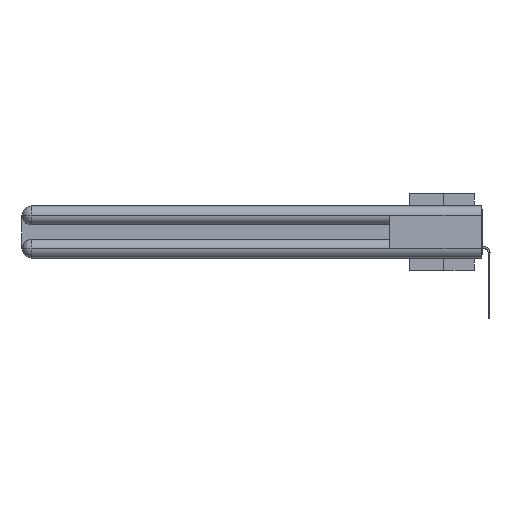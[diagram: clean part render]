
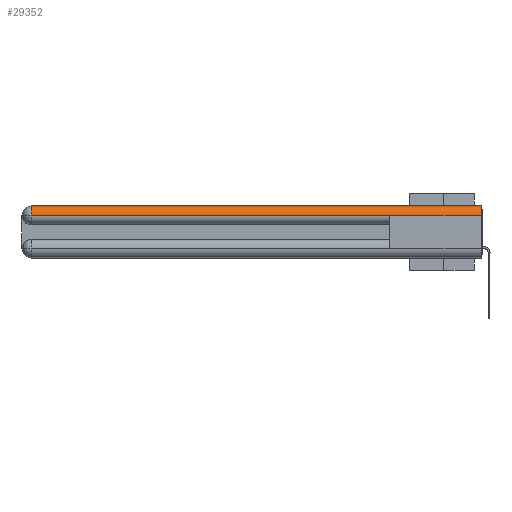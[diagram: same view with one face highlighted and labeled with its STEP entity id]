
A CAD part, left-side view. The second image highlights one B-rep face of the part: STEP entity #29352.
In plain terms, the highlighted cylindrical face has radius 1.562 mm (diameter 3.124 mm), a partial arc.
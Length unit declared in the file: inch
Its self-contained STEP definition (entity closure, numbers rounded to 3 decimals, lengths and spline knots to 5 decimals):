
#636 = LINE ( 'NONE', #3860, #15750 ) ;
#1578 = DIRECTION ( 'NONE',  ( 0., 0., 1. ) ) ;
#1835 = AXIS2_PLACEMENT_3D ( 'NONE', #13477, #21405, #1578 ) ;
#2423 = EDGE_LOOP ( 'NONE', ( #30328, #17633, #7823, #13776, #29750 ) ) ;
#3426 = DIRECTION ( 'NONE',  ( 1., 0., 0. ) ) ;
#3727 = CARTESIAN_POINT ( 'NONE',  ( 0., 3., -0.0615 ) ) ;
#3860 = CARTESIAN_POINT ( 'NONE',  ( 0.0615, 0., 0. ) ) ;
#4786 = VECTOR ( 'NONE', #35011, 39.37008 ) ;
#6468 = VECTOR ( 'NONE', #12490, 39.37008 ) ;
#6993 = VERTEX_POINT ( 'NONE', #33838 ) ;
#7823 = ORIENTED_EDGE ( 'NONE', *, *, #29557, .T. ) ;
#9452 = CARTESIAN_POINT ( 'NONE',  ( 0.0615, 0., -0.0615 ) ) ;
#10707 = CARTESIAN_POINT ( 'NONE',  ( 0., 2.94, -0.0615 ) ) ;
#12222 = LINE ( 'NONE', #3727, #4786 ) ;
#12490 = DIRECTION ( 'NONE',  ( 0., 1., 0. ) ) ;
#13162 = CIRCLE ( 'NONE', #34197, 0.0615 ) ;
#13477 = CARTESIAN_POINT ( 'NONE',  ( 0.0615, 2.94, -0.0615 ) ) ;
#13558 = VERTEX_POINT ( 'NONE', #17473 ) ;
#13776 = ORIENTED_EDGE ( 'NONE', *, *, #15268, .F. ) ;
#15144 = LINE ( 'NONE', #35475, #6468 ) ;
#15268 = EDGE_CURVE ( 'NONE', #6993, #36753, #15144, .T. ) ;
#15746 = DIRECTION ( 'NONE',  ( 0., -1., 0. ) ) ;
#15750 = VECTOR ( 'NONE', #15746, 39.37008 ) ;
#16899 = CIRCLE ( 'NONE', #1835, 0.0615 ) ;
#17440 = AXIS2_PLACEMENT_3D ( 'NONE', #26167, #29166, #17526 ) ;
#17473 = CARTESIAN_POINT ( 'NONE',  ( 0.0615, 0., 0. ) ) ;
#17526 = DIRECTION ( 'NONE',  ( 0., 0., 1. ) ) ;
#17633 = ORIENTED_EDGE ( 'NONE', *, *, #36425, .T. ) ;
#20985 = CARTESIAN_POINT ( 'NONE',  ( 0., 0.6, -0.0615 ) ) ;
#21405 = DIRECTION ( 'NONE',  ( 0., -1., 0. ) ) ;
#25004 = VERTEX_POINT ( 'NONE', #31355 ) ;
#25607 = CYLINDRICAL_SURFACE ( 'NONE', #17440, 0.0615 ) ;
#26167 = CARTESIAN_POINT ( 'NONE',  ( 0.0615, 0., -0.0615 ) ) ;
#29166 = DIRECTION ( 'NONE',  ( 0., 1., 0. ) ) ;
#29352 = ADVANCED_FACE ( 'NONE', ( #31610 ), #25607, .T. ) ;
#29557 = EDGE_CURVE ( 'NONE', #33645, #36753, #12222, .T. ) ;
#29750 = ORIENTED_EDGE ( 'NONE', *, *, #32968, .F. ) ;
#30328 = ORIENTED_EDGE ( 'NONE', *, *, #35737, .F. ) ;
#31355 = CARTESIAN_POINT ( 'NONE',  ( 0.0615, 2.94, 0. ) ) ;
#31610 = FACE_OUTER_BOUND ( 'NONE', #2423, .T. ) ;
#32968 = EDGE_CURVE ( 'NONE', #13558, #6993, #13162, .T. ) ;
#33645 = VERTEX_POINT ( 'NONE', #10707 ) ;
#33838 = CARTESIAN_POINT ( 'NONE',  ( 0., 0., -0.0615 ) ) ;
#34197 = AXIS2_PLACEMENT_3D ( 'NONE', #9452, #35089, #3426 ) ;
#35011 = DIRECTION ( 'NONE',  ( 0., -1., 0. ) ) ;
#35089 = DIRECTION ( 'NONE',  ( 0., -1., 0. ) ) ;
#35475 = CARTESIAN_POINT ( 'NONE',  ( 0., 3., -0.0615 ) ) ;
#35737 = EDGE_CURVE ( 'NONE', #25004, #13558, #636, .T. ) ;
#36425 = EDGE_CURVE ( 'NONE', #25004, #33645, #16899, .T. ) ;
#36753 = VERTEX_POINT ( 'NONE', #20985 ) ;
